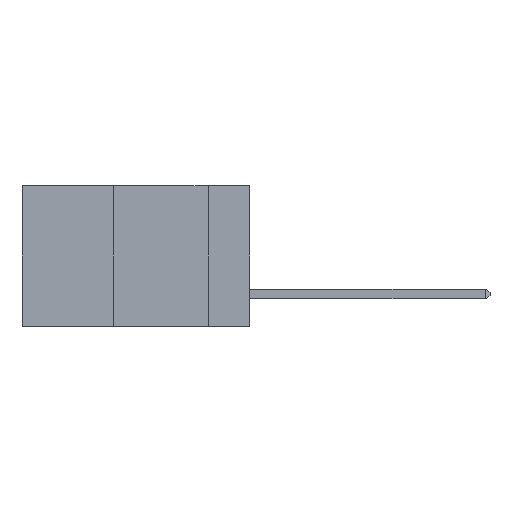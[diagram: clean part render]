
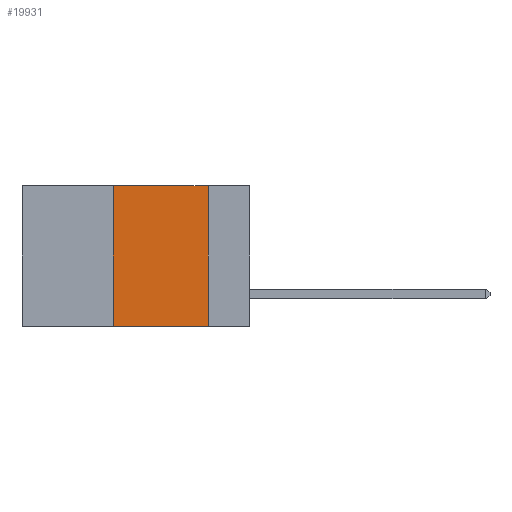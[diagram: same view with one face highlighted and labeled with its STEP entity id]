
A CAD part, left-side view. The second image highlights one B-rep face of the part: STEP entity #19931.
In plain terms, the highlighted planar face has unit normal (-1, 0, 0).
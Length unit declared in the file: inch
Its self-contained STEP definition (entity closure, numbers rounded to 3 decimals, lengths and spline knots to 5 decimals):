
#1038 = VERTEX_POINT ( 'NONE', #20046 ) ;
#1638 = ORIENTED_EDGE ( 'NONE', *, *, #4255, .F. ) ;
#2063 = VERTEX_POINT ( 'NONE', #16009 ) ;
#2292 = DIRECTION ( 'NONE',  ( 0., -1., 0. ) ) ;
#2299 = DIRECTION ( 'NONE',  ( 1., 0., 0. ) ) ;
#2349 = DIRECTION ( 'NONE',  ( 0., 0., 1. ) ) ;
#2405 = CARTESIAN_POINT ( 'NONE',  ( 0., 0.36, -0.37 ) ) ;
#2429 = VERTEX_POINT ( 'NONE', #2405 ) ;
#3033 = EDGE_CURVE ( 'NONE', #2429, #5856, #17198, .T. ) ;
#4255 = EDGE_CURVE ( 'NONE', #2429, #1038, #10695, .T. ) ;
#5856 = VERTEX_POINT ( 'NONE', #11157 ) ;
#7523 = FACE_OUTER_BOUND ( 'NONE', #17416, .T. ) ;
#8463 = DIRECTION ( 'NONE',  ( 0., -1., 0. ) ) ;
#9026 = ORIENTED_EDGE ( 'NONE', *, *, #3033, .T. ) ;
#9212 = EDGE_CURVE ( 'NONE', #2063, #5856, #13424, .T. ) ;
#10224 = CARTESIAN_POINT ( 'NONE',  ( 0., 0.6, 0. ) ) ;
#10695 = LINE ( 'NONE', #11601, #20242 ) ;
#11028 = VECTOR ( 'NONE', #8463, 39.37008 ) ;
#11157 = CARTESIAN_POINT ( 'NONE',  ( 0., 0.11, -0.37 ) ) ;
#11601 = CARTESIAN_POINT ( 'NONE',  ( 0., 0.36, 0. ) ) ;
#12332 = EDGE_CURVE ( 'NONE', #1038, #2063, #15831, .T. ) ;
#13288 = CARTESIAN_POINT ( 'NONE',  ( 0., 0.6, 0. ) ) ;
#13424 = LINE ( 'NONE', #21124, #22414 ) ;
#15115 = DIRECTION ( 'NONE',  ( 0., 0., -1. ) ) ;
#15831 = LINE ( 'NONE', #10224, #11028 ) ;
#16009 = CARTESIAN_POINT ( 'NONE',  ( 0., 0.11, 0. ) ) ;
#16685 = DIRECTION ( 'NONE',  ( 0., 0., -1. ) ) ;
#17198 = LINE ( 'NONE', #22231, #17756 ) ;
#17258 = ORIENTED_EDGE ( 'NONE', *, *, #12332, .F. ) ;
#17416 = EDGE_LOOP ( 'NONE', ( #20606, #17258, #1638, #9026 ) ) ;
#17756 = VECTOR ( 'NONE', #2292, 39.37008 ) ;
#19757 = AXIS2_PLACEMENT_3D ( 'NONE', #13288, #2299, #15115 ) ;
#19931 = ADVANCED_FACE ( 'NONE', ( #7523 ), #20443, .F. ) ;
#20046 = CARTESIAN_POINT ( 'NONE',  ( 0., 0.36, 0. ) ) ;
#20242 = VECTOR ( 'NONE', #2349, 39.37008 ) ;
#20443 = PLANE ( 'NONE',  #19757 ) ;
#20606 = ORIENTED_EDGE ( 'NONE', *, *, #9212, .F. ) ;
#21124 = CARTESIAN_POINT ( 'NONE',  ( 0., 0.11, 0. ) ) ;
#22231 = CARTESIAN_POINT ( 'NONE',  ( 0., 0.6, -0.37 ) ) ;
#22414 = VECTOR ( 'NONE', #16685, 39.37008 ) ;
